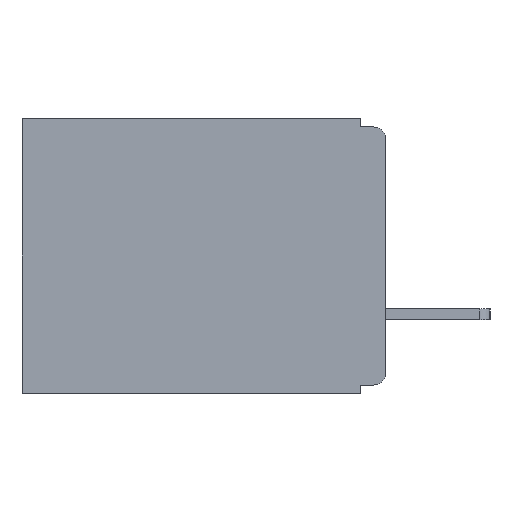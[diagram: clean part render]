
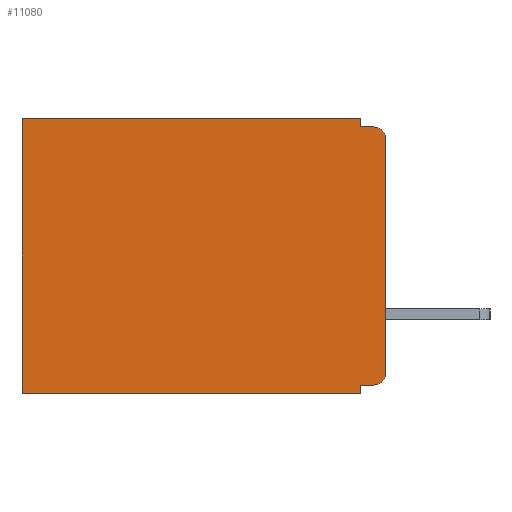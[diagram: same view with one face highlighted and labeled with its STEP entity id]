
A CAD part, left-side view. The second image highlights one B-rep face of the part: STEP entity #11080.
In plain terms, the highlighted planar face has unit normal (-1, 0, 0).
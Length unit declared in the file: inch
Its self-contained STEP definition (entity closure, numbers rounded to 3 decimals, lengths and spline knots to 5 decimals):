
#199 = DIRECTION ( 'NONE',  ( -1., 0., 0. ) ) ;
#676 = CARTESIAN_POINT ( 'NONE',  ( 0.3, 0., -0.025 ) ) ;
#780 = ORIENTED_EDGE ( 'NONE', *, *, #3395, .F. ) ;
#906 = DIRECTION ( 'NONE',  ( 1., 0., 0. ) ) ;
#966 = LINE ( 'NONE', #8520, #14032 ) ;
#1015 = CARTESIAN_POINT ( 'NONE',  ( 0.3, 0.031, 0. ) ) ;
#1482 = CARTESIAN_POINT ( 'NONE',  ( 0.3, 0.031, -0.01 ) ) ;
#2018 = VECTOR ( 'NONE', #22133, 39.37008 ) ;
#2071 = ORIENTED_EDGE ( 'NONE', *, *, #4312, .F. ) ;
#2306 = DIRECTION ( 'NONE',  ( 0., 1., 0. ) ) ;
#2532 = AXIS2_PLACEMENT_3D ( 'NONE', #12006, #906, #13894 ) ;
#2627 = EDGE_CURVE ( 'NONE', #17706, #23048, #6754, .T. ) ;
#3395 = EDGE_CURVE ( 'NONE', #17830, #17706, #17746, .T. ) ;
#3526 = VECTOR ( 'NONE', #6270, 39.37008 ) ;
#3705 = DIRECTION ( 'NONE',  ( 0., -1., 0. ) ) ;
#4312 = EDGE_CURVE ( 'NONE', #14495, #18700, #12758, .T. ) ;
#4485 = EDGE_CURVE ( 'NONE', #14495, #21180, #11850, .T. ) ;
#4609 = LINE ( 'NONE', #22326, #18251 ) ;
#5545 = EDGE_CURVE ( 'NONE', #11644, #11875, #8089, .T. ) ;
#5595 = VECTOR ( 'NONE', #18499, 39.37008 ) ;
#5700 = EDGE_CURVE ( 'NONE', #18700, #13798, #4609, .T. ) ;
#6254 = CARTESIAN_POINT ( 'NONE',  ( 0.3, 0.015, -0.01 ) ) ;
#6270 = DIRECTION ( 'NONE',  ( 0., 0., -1. ) ) ;
#6623 = DIRECTION ( 'NONE',  ( -1., 0., 0. ) ) ;
#6712 = ORIENTED_EDGE ( 'NONE', *, *, #16386, .T. ) ;
#6754 = LINE ( 'NONE', #20300, #5595 ) ;
#6796 = ORIENTED_EDGE ( 'NONE', *, *, #4485, .T. ) ;
#7295 = CARTESIAN_POINT ( 'NONE',  ( 0.3, 0.437, 0. ) ) ;
#7991 = EDGE_LOOP ( 'NONE', ( #11385, #6712, #10862, #2071, #6796, #21223, #13177, #780, #16370, #23500 ) ) ;
#8089 = CIRCLE ( 'NONE', #22104, 0.015 ) ;
#8168 = CARTESIAN_POINT ( 'NONE',  ( 0.3, 0.437, -0.33 ) ) ;
#8520 = CARTESIAN_POINT ( 'NONE',  ( 0.3, 0., -0.33 ) ) ;
#9448 = EDGE_CURVE ( 'NONE', #11644, #17830, #22153, .T. ) ;
#10862 = ORIENTED_EDGE ( 'NONE', *, *, #5700, .F. ) ;
#11080 = ADVANCED_FACE ( 'NONE', ( #14468 ), #19446, .F. ) ;
#11284 = CARTESIAN_POINT ( 'NONE',  ( 0.3, 0.015, -0.025 ) ) ;
#11330 = LINE ( 'NONE', #14384, #20115 ) ;
#11385 = ORIENTED_EDGE ( 'NONE', *, *, #19138, .F. ) ;
#11644 = VERTEX_POINT ( 'NONE', #17353 ) ;
#11850 = LINE ( 'NONE', #16500, #2018 ) ;
#11875 = VERTEX_POINT ( 'NONE', #14416 ) ;
#12006 = CARTESIAN_POINT ( 'NONE',  ( 0.3, 0., -0.33 ) ) ;
#12260 = CARTESIAN_POINT ( 'NONE',  ( 0.3, 0.031, 0. ) ) ;
#12758 = LINE ( 'NONE', #12260, #17120 ) ;
#13177 = ORIENTED_EDGE ( 'NONE', *, *, #2627, .F. ) ;
#13186 = DIRECTION ( 'NONE',  ( 0., 0., -1. ) ) ;
#13311 = CIRCLE ( 'NONE', #23910, 0.015 ) ;
#13798 = VERTEX_POINT ( 'NONE', #6254 ) ;
#13894 = DIRECTION ( 'NONE',  ( 0., 0., -1. ) ) ;
#14032 = VECTOR ( 'NONE', #19675, 39.37008 ) ;
#14144 = DIRECTION ( 'NONE',  ( 0., 0., -1. ) ) ;
#14384 = CARTESIAN_POINT ( 'NONE',  ( 0.3, 0.437, -0.33 ) ) ;
#14416 = CARTESIAN_POINT ( 'NONE',  ( 0.3, 0., -0.305 ) ) ;
#14468 = FACE_OUTER_BOUND ( 'NONE', #7991, .T. ) ;
#14495 = VERTEX_POINT ( 'NONE', #1015 ) ;
#16258 = DIRECTION ( 'NONE',  ( 0., 0., -1. ) ) ;
#16370 = ORIENTED_EDGE ( 'NONE', *, *, #9448, .F. ) ;
#16386 = EDGE_CURVE ( 'NONE', #18453, #13798, #13311, .T. ) ;
#16500 = CARTESIAN_POINT ( 'NONE',  ( 0.3, 0., 0. ) ) ;
#17120 = VECTOR ( 'NONE', #14144, 39.37008 ) ;
#17353 = CARTESIAN_POINT ( 'NONE',  ( 0.3, 0.015, -0.32 ) ) ;
#17706 = VERTEX_POINT ( 'NONE', #22664 ) ;
#17744 = CARTESIAN_POINT ( 'NONE',  ( 0.3, 0.015, -0.305 ) ) ;
#17746 = LINE ( 'NONE', #23038, #3526 ) ;
#17830 = VERTEX_POINT ( 'NONE', #19323 ) ;
#18251 = VECTOR ( 'NONE', #3705, 39.37008 ) ;
#18453 = VERTEX_POINT ( 'NONE', #676 ) ;
#18499 = DIRECTION ( 'NONE',  ( 0., 1., 0. ) ) ;
#18700 = VERTEX_POINT ( 'NONE', #1482 ) ;
#18968 = CARTESIAN_POINT ( 'NONE',  ( 0.3, 0., -0.32 ) ) ;
#19138 = EDGE_CURVE ( 'NONE', #18453, #11875, #966, .T. ) ;
#19323 = CARTESIAN_POINT ( 'NONE',  ( 0.3, 0.031, -0.32 ) ) ;
#19446 = PLANE ( 'NONE',  #2532 ) ;
#19643 = DIRECTION ( 'NONE',  ( 0., 0., -1. ) ) ;
#19675 = DIRECTION ( 'NONE',  ( 0., 0., -1. ) ) ;
#20115 = VECTOR ( 'NONE', #16258, 39.37008 ) ;
#20300 = CARTESIAN_POINT ( 'NONE',  ( 0.3, 0., -0.33 ) ) ;
#20467 = EDGE_CURVE ( 'NONE', #21180, #23048, #11330, .T. ) ;
#21180 = VERTEX_POINT ( 'NONE', #7295 ) ;
#21223 = ORIENTED_EDGE ( 'NONE', *, *, #20467, .T. ) ;
#21563 = VECTOR ( 'NONE', #2306, 39.37008 ) ;
#22104 = AXIS2_PLACEMENT_3D ( 'NONE', #17744, #6623, #19643 ) ;
#22133 = DIRECTION ( 'NONE',  ( 0., 1., 0. ) ) ;
#22153 = LINE ( 'NONE', #18968, #21563 ) ;
#22326 = CARTESIAN_POINT ( 'NONE',  ( 0.3, 0., -0.01 ) ) ;
#22664 = CARTESIAN_POINT ( 'NONE',  ( 0.3, 0.031, -0.33 ) ) ;
#23038 = CARTESIAN_POINT ( 'NONE',  ( 0.3, 0.031, -0.33 ) ) ;
#23048 = VERTEX_POINT ( 'NONE', #8168 ) ;
#23500 = ORIENTED_EDGE ( 'NONE', *, *, #5545, .T. ) ;
#23910 = AXIS2_PLACEMENT_3D ( 'NONE', #11284, #199, #13186 ) ;
